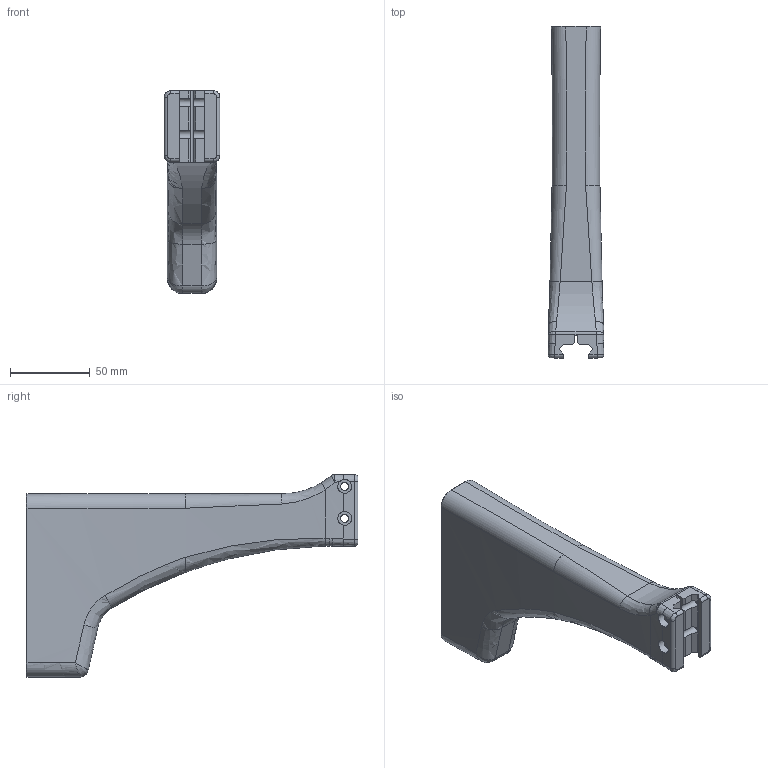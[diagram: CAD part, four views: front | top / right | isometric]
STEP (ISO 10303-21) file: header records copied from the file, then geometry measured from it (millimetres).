
FILE_DESCRIPTION(/* description */ (''),/* implementation_level */ '2;1');
FILE_NAME(/* name */ 'Single Print.step',/* time_stamp */ '2021-07-28T09:04:31-04:00',/* author */ (''),/* organization */ (''),/* preprocessor_version */ 'ST-DEVELOPER v18.1',/* originating_system */ 'Autodesk Translation Framework v10.9.0.1377',/* authorisation */ '');
FILE_SCHEMA (('AUTOMOTIVE_DESIGN { 1 0 10303 214 3 1 1 }'));
Length unit declared in the file: millimetre
Products named in the file (1): Single Print
Bounding box: 35 x 208.01 x 127 mm (x, y, z)
Volume: 216776.4 mm3; surface area: 66786.6 mm2
Topology: 1 solids, 2 shells, 253 faces, 673 edges, 408 vertices
Faces by surface type: bspline 103, plane 81, cylinder 45, torus 22, cone 2
Full cylindrical faces by diameter (mm): 4 x2, 5.1 x4, 8.75 x2
Entity records: 11796 total; most frequent: CARTESIAN_POINT 6208, ORIENTED_EDGE 1314, DIRECTION 909, EDGE_CURVE 657, VERTEX_POINT 408, AXIS2_PLACEMENT_3D 342, EDGE_LOOP 265, FACE_OUTER_BOUND 253
